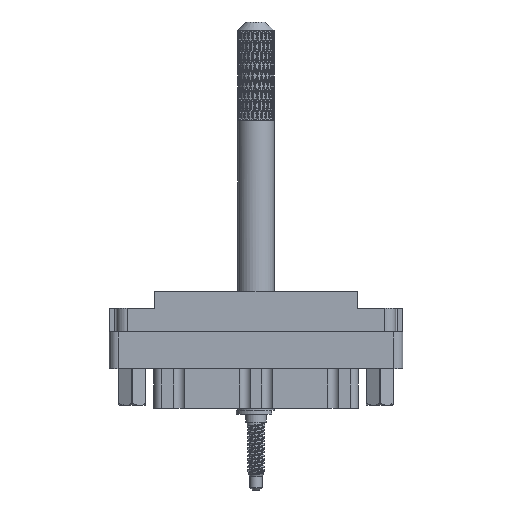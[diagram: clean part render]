
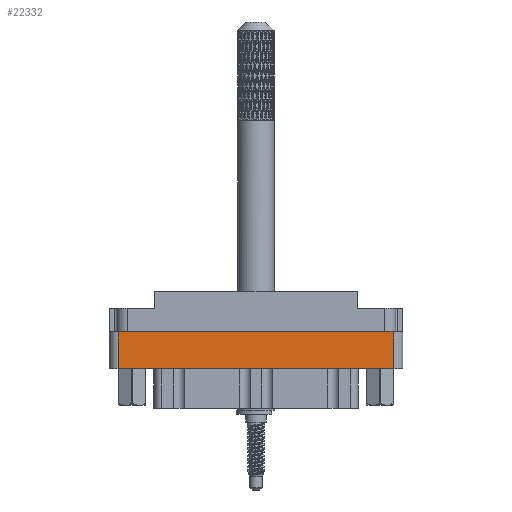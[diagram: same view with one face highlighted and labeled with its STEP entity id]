
A CAD part, front view. The second image highlights one B-rep face of the part: STEP entity #22332.
In plain terms, the highlighted planar face has unit normal (0, -1, 0).
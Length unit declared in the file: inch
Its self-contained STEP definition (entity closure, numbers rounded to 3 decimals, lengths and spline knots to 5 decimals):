
#2177 = LINE ( 'NONE', #42211, #99656 ) ;
#5283 = CARTESIAN_POINT ( 'NONE',  ( 0.938, -0.438, -0.529 ) ) ;
#7617 = VERTEX_POINT ( 'NONE', #90599 ) ;
#8388 = DIRECTION ( 'NONE',  ( 0., 0., -1. ) ) ;
#8819 = EDGE_CURVE ( 'NONE', #79531, #7617, #100801, .T. ) ;
#9414 = CARTESIAN_POINT ( 'NONE',  ( -0.938, -0.438, -0.798 ) ) ;
#16429 = DIRECTION ( 'NONE',  ( -1., 0., 0. ) ) ;
#21702 = EDGE_CURVE ( 'NONE', #105855, #22663, #105314, .T. ) ;
#22332 = ADVANCED_FACE ( 'NONE', ( #83553 ), #24604, .T. ) ;
#22663 = VERTEX_POINT ( 'NONE', #35069 ) ;
#24604 = PLANE ( 'NONE',  #77436 ) ;
#29577 = DIRECTION ( 'NONE',  ( 0., 0., 1. ) ) ;
#33512 = EDGE_CURVE ( 'NONE', #79531, #22663, #58836, .T. ) ;
#35069 = CARTESIAN_POINT ( 'NONE',  ( 0.938, -0.438, -0.277 ) ) ;
#42211 = CARTESIAN_POINT ( 'NONE',  ( -0.938, -0.438, -0.798 ) ) ;
#45009 = ORIENTED_EDGE ( 'NONE', *, *, #21702, .F. ) ;
#49986 = CARTESIAN_POINT ( 'NONE',  ( 0.938, -0.438, -0.529 ) ) ;
#56862 = EDGE_LOOP ( 'NONE', ( #90429, #64744, #100336, #45009 ) ) ;
#58836 = LINE ( 'NONE', #91834, #71771 ) ;
#64744 = ORIENTED_EDGE ( 'NONE', *, *, #8819, .F. ) ;
#67505 = VECTOR ( 'NONE', #16429, 39.37008 ) ;
#71771 = VECTOR ( 'NONE', #29577, 39.37008 ) ;
#75272 = DIRECTION ( 'NONE',  ( 0., 0., 1. ) ) ;
#77436 = AXIS2_PLACEMENT_3D ( 'NONE', #9414, #82521, #8388 ) ;
#79531 = VERTEX_POINT ( 'NONE', #5283 ) ;
#82521 = DIRECTION ( 'NONE',  ( 0., -1., 0. ) ) ;
#83553 = FACE_OUTER_BOUND ( 'NONE', #56862, .T. ) ;
#86375 = CARTESIAN_POINT ( 'NONE',  ( -0.938, -0.438, -0.277 ) ) ;
#90124 = CARTESIAN_POINT ( 'NONE',  ( -1., -0.438, -0.277 ) ) ;
#90429 = ORIENTED_EDGE ( 'NONE', *, *, #99172, .F. ) ;
#90599 = CARTESIAN_POINT ( 'NONE',  ( -0.938, -0.438, -0.529 ) ) ;
#91170 = DIRECTION ( 'NONE',  ( 1., 0., 0. ) ) ;
#91834 = CARTESIAN_POINT ( 'NONE',  ( 0.938, -0.438, -0.798 ) ) ;
#96536 = VECTOR ( 'NONE', #91170, 39.37008 ) ;
#99172 = EDGE_CURVE ( 'NONE', #7617, #105855, #2177, .T. ) ;
#99656 = VECTOR ( 'NONE', #75272, 39.37008 ) ;
#100336 = ORIENTED_EDGE ( 'NONE', *, *, #33512, .T. ) ;
#100801 = LINE ( 'NONE', #49986, #67505 ) ;
#105314 = LINE ( 'NONE', #90124, #96536 ) ;
#105855 = VERTEX_POINT ( 'NONE', #86375 ) ;
